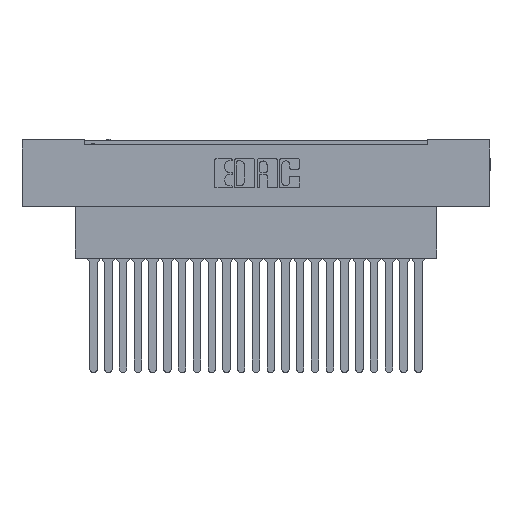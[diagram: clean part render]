
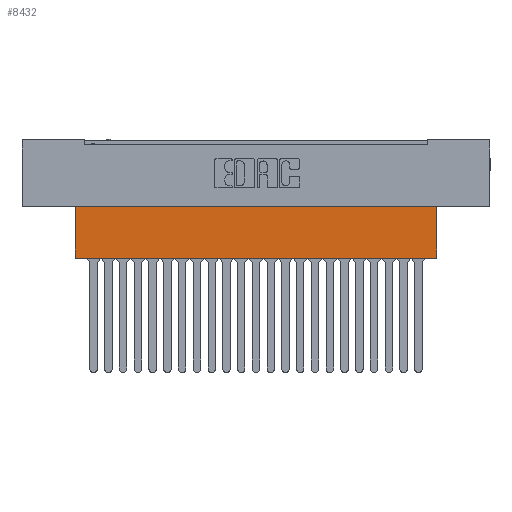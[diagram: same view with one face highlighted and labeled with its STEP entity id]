
A CAD part, top view. The second image highlights one B-rep face of the part: STEP entity #8432.
In plain terms, the highlighted planar face has unit normal (0, 0, 1).
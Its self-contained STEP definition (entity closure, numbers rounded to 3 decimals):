
#433 = VERTEX_POINT ( 'NONE', #27295 ) ;
#654 = DIRECTION ( 'NONE',  ( -1., 0., 0. ) ) ;
#1323 = EDGE_CURVE ( 'NONE', #22481, #18461, #9292, .T. ) ;
#1659 = AXIS2_PLACEMENT_3D ( 'NONE', #23387, #11666, #27879 ) ;
#1740 = LINE ( 'NONE', #22561, #27280 ) ;
#1742 = EDGE_LOOP ( 'NONE', ( #23289, #16560, #10064, #5465 ) ) ;
#2613 = VECTOR ( 'NONE', #6296, 1000. ) ;
#4991 = VECTOR ( 'NONE', #6065, 1000. ) ;
#5375 = CARTESIAN_POINT ( 'NONE',  ( 80.518, 0., -3.962 ) ) ;
#5465 = ORIENTED_EDGE ( 'NONE', *, *, #1323, .F. ) ;
#6065 = DIRECTION ( 'NONE',  ( 0., 1., 0. ) ) ;
#6296 = DIRECTION ( 'NONE',  ( -1., 0., 0. ) ) ;
#6412 = VERTEX_POINT ( 'NONE', #18138 ) ;
#8432 = ADVANCED_FACE ( 'NONE', ( #15469 ), #15994, .F. ) ;
#8680 = CARTESIAN_POINT ( 'NONE',  ( 80.518, -8.814, -3.962 ) ) ;
#9292 = LINE ( 'NONE', #15078, #4991 ) ;
#10064 = ORIENTED_EDGE ( 'NONE', *, *, #16511, .T. ) ;
#11666 = DIRECTION ( 'NONE',  ( 0., 0., -1. ) ) ;
#15078 = CARTESIAN_POINT ( 'NONE',  ( 9.144, -8.814, -3.962 ) ) ;
#15469 = FACE_OUTER_BOUND ( 'NONE', #1742, .T. ) ;
#15994 = PLANE ( 'NONE',  #1659 ) ;
#16511 = EDGE_CURVE ( 'NONE', #6412, #18461, #28403, .T. ) ;
#16560 = ORIENTED_EDGE ( 'NONE', *, *, #18282, .F. ) ;
#18138 = CARTESIAN_POINT ( 'NONE',  ( 71.374, 0., -3.962 ) ) ;
#18282 = EDGE_CURVE ( 'NONE', #6412, #433, #1740, .T. ) ;
#18461 = VERTEX_POINT ( 'NONE', #23054 ) ;
#19493 = LINE ( 'NONE', #8680, #2613 ) ;
#20979 = CARTESIAN_POINT ( 'NONE',  ( 9.144, -8.814, -3.962 ) ) ;
#22481 = VERTEX_POINT ( 'NONE', #20979 ) ;
#22561 = CARTESIAN_POINT ( 'NONE',  ( 71.374, -8.814, -3.962 ) ) ;
#23054 = CARTESIAN_POINT ( 'NONE',  ( 9.144, 0., -3.962 ) ) ;
#23289 = ORIENTED_EDGE ( 'NONE', *, *, #26726, .F. ) ;
#23387 = CARTESIAN_POINT ( 'NONE',  ( 80.518, 0., -3.962 ) ) ;
#23762 = VECTOR ( 'NONE', #654, 1000. ) ;
#26726 = EDGE_CURVE ( 'NONE', #433, #22481, #19493, .T. ) ;
#27280 = VECTOR ( 'NONE', #29451, 1000. ) ;
#27295 = CARTESIAN_POINT ( 'NONE',  ( 71.374, -8.814, -3.962 ) ) ;
#27879 = DIRECTION ( 'NONE',  ( 0., 1., 0. ) ) ;
#28403 = LINE ( 'NONE', #5375, #23762 ) ;
#29451 = DIRECTION ( 'NONE',  ( 0., -1., 0. ) ) ;
